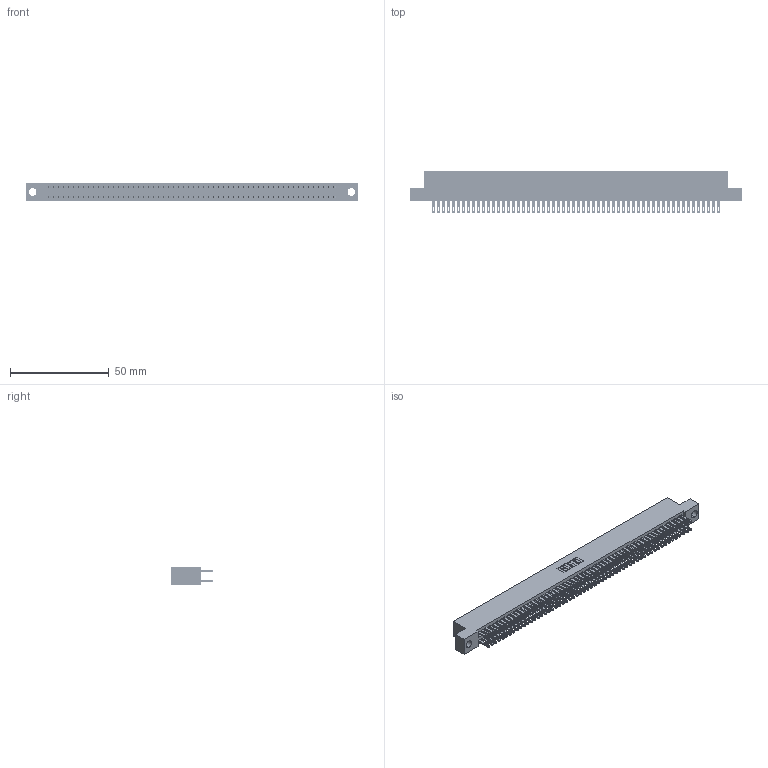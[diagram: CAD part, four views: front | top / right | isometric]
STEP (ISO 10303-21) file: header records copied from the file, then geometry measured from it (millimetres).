
FILE_DESCRIPTION (( 'STEP AP203' ), '1' );
FILE_NAME ('895-116-500-204.STEP', '2020-10-13T14:10:00', ( '' ), ( '' ), 'SwSTEP 2.0', 'SolidWorks 2020', '' );
FILE_SCHEMA (( 'CONFIG_CONTROL_DESIGN' ));
Length unit declared in the file: inch
Products named in the file (3): 895-116-500-204; 345-292-001_345-293-100; 845 Part_Flush Mounting Lugs - 0.156 Dia-TH
Assembly tree (117 placements, depth 2):
  895-116-500-204
    845 Part_Flush Mounting Lugs - 0.156 Dia-TH
    345-292-001_345-293-100  x116
Bounding box: 168.53 x 21.51 x 9.4 mm (x, y, z)
Volume: 16786.2 mm3; surface area: 26121 mm2
Topology: 117 solids, 117 shells, 5462 faces, 16697 edges, 11130 vertices
Faces by surface type: plane 3212, cylinder 2250
Entity records: 43287 total; most frequent: CARTESIAN_POINT 7240, ORIENTED_EDGE 7174, DIRECTION 6367, EDGE_CURVE 3587, LINE 3219, VECTOR 3219, VERTEX_POINT 2390, AXIS2_PLACEMENT_3D 1574
